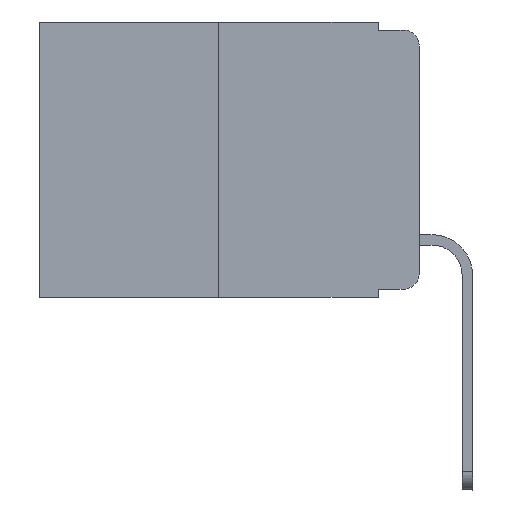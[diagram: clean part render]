
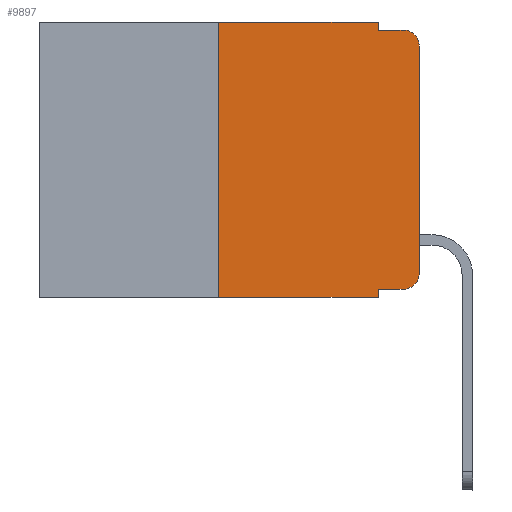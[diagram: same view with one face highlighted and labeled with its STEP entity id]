
A CAD part, left-side view. The second image highlights one B-rep face of the part: STEP entity #9897.
In plain terms, the highlighted planar face has unit normal (-1, 0, 0).
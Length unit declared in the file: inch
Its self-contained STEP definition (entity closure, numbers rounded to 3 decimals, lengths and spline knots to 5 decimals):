
#70 = DIRECTION ( 'NONE',  ( 0., 0., -1. ) ) ;
#277 = VERTEX_POINT ( 'NONE', #10054 ) ;
#329 = LINE ( 'NONE', #1274, #8766 ) ;
#504 = CARTESIAN_POINT ( 'NONE',  ( 0., 0.051, -0.333 ) ) ;
#809 = ORIENTED_EDGE ( 'NONE', *, *, #3885, .T. ) ;
#959 = LINE ( 'NONE', #3581, #6711 ) ;
#1002 = CARTESIAN_POINT ( 'NONE',  ( 0., 0.02, -0.01 ) ) ;
#1059 = VERTEX_POINT ( 'NONE', #4307 ) ;
#1081 = DIRECTION ( 'NONE',  ( 0., -1., 0. ) ) ;
#1229 = LINE ( 'NONE', #7632, #9691 ) ;
#1274 = CARTESIAN_POINT ( 'NONE',  ( 0., 0.051, 0. ) ) ;
#1391 = DIRECTION ( 'NONE',  ( 1., 0., 0. ) ) ;
#1441 = CARTESIAN_POINT ( 'NONE',  ( 0., 0.051, -0.333 ) ) ;
#1515 = EDGE_CURVE ( 'NONE', #10749, #10752, #8075, .T. ) ;
#1640 = ORIENTED_EDGE ( 'NONE', *, *, #2505, .F. ) ;
#1793 = ORIENTED_EDGE ( 'NONE', *, *, #2045, .T. ) ;
#1835 = CARTESIAN_POINT ( 'NONE',  ( 0., 0., -0.03 ) ) ;
#1882 = EDGE_LOOP ( 'NONE', ( #5099, #2190, #9951, #11490, #10899, #3770, #1793, #1640, #809, #9549 ) ) ;
#2009 = DIRECTION ( 'NONE',  ( 0., 0., -1. ) ) ;
#2045 = EDGE_CURVE ( 'NONE', #7577, #7876, #5255, .T. ) ;
#2190 = ORIENTED_EDGE ( 'NONE', *, *, #1515, .T. ) ;
#2258 = LINE ( 'NONE', #504, #5525 ) ;
#2370 = CARTESIAN_POINT ( 'NONE',  ( 0., 0.051, -0.343 ) ) ;
#2505 = EDGE_CURVE ( 'NONE', #11327, #7876, #9865, .T. ) ;
#2786 = CARTESIAN_POINT ( 'NONE',  ( 0., 0.051, -0.01 ) ) ;
#2829 = DIRECTION ( 'NONE',  ( 0., 0., -1. ) ) ;
#2870 = VECTOR ( 'NONE', #6007, 39.37008 ) ;
#3147 = PLANE ( 'NONE',  #6907 ) ;
#3581 = CARTESIAN_POINT ( 'NONE',  ( 0., 0., 0. ) ) ;
#3628 = CARTESIAN_POINT ( 'NONE',  ( 0., 0.051, 0. ) ) ;
#3770 = ORIENTED_EDGE ( 'NONE', *, *, #8933, .F. ) ;
#3787 = CARTESIAN_POINT ( 'NONE',  ( 0., 0.25, -0.343 ) ) ;
#3885 = EDGE_CURVE ( 'NONE', #11327, #277, #2258, .T. ) ;
#4074 = DIRECTION ( 'NONE',  ( 0., -1., 0. ) ) ;
#4307 = CARTESIAN_POINT ( 'NONE',  ( 0., 0.25, 0. ) ) ;
#4367 = EDGE_CURVE ( 'NONE', #10366, #10752, #10972, .T. ) ;
#4711 = EDGE_CURVE ( 'NONE', #277, #7251, #8135, .T. ) ;
#4944 = CARTESIAN_POINT ( 'NONE',  ( 0., 0.051, 0. ) ) ;
#5099 = ORIENTED_EDGE ( 'NONE', *, *, #9207, .T. ) ;
#5255 = LINE ( 'NONE', #6184, #10848 ) ;
#5421 = DIRECTION ( 'NONE',  ( 0., 0., 1. ) ) ;
#5525 = VECTOR ( 'NONE', #4074, 39.37008 ) ;
#5894 = CARTESIAN_POINT ( 'NONE',  ( 0., 0.473, 0. ) ) ;
#6007 = DIRECTION ( 'NONE',  ( 0., -1., 0. ) ) ;
#6184 = CARTESIAN_POINT ( 'NONE',  ( 0., 0.473, -0.343 ) ) ;
#6367 = DIRECTION ( 'NONE',  ( -1., 0., 0. ) ) ;
#6380 = DIRECTION ( 'NONE',  ( 0., -1., 0. ) ) ;
#6408 = CARTESIAN_POINT ( 'NONE',  ( 0., 0.02, -0.03 ) ) ;
#6418 = CARTESIAN_POINT ( 'NONE',  ( 0., 0., -0.313 ) ) ;
#6455 = EDGE_CURVE ( 'NONE', #1059, #9438, #7382, .T. ) ;
#6711 = VECTOR ( 'NONE', #5421, 39.37008 ) ;
#6907 = AXIS2_PLACEMENT_3D ( 'NONE', #7692, #1391, #9592 ) ;
#7000 = AXIS2_PLACEMENT_3D ( 'NONE', #10849, #6367, #2829 ) ;
#7251 = VERTEX_POINT ( 'NONE', #6418 ) ;
#7382 = LINE ( 'NONE', #5894, #2870 ) ;
#7577 = VERTEX_POINT ( 'NONE', #3787 ) ;
#7632 = CARTESIAN_POINT ( 'NONE',  ( 0., 0.25, 0. ) ) ;
#7692 = CARTESIAN_POINT ( 'NONE',  ( 0., 0.473, 0. ) ) ;
#7758 = VECTOR ( 'NONE', #9752, 39.37008 ) ;
#7876 = VERTEX_POINT ( 'NONE', #2370 ) ;
#8075 = CIRCLE ( 'NONE', #8438, 0.02 ) ;
#8135 = CIRCLE ( 'NONE', #7000, 0.02 ) ;
#8438 = AXIS2_PLACEMENT_3D ( 'NONE', #6408, #11000, #2009 ) ;
#8474 = CARTESIAN_POINT ( 'NONE',  ( 0., 0.051, -0.01 ) ) ;
#8658 = EDGE_CURVE ( 'NONE', #9438, #10366, #329, .T. ) ;
#8766 = VECTOR ( 'NONE', #70, 39.37008 ) ;
#8801 = FACE_OUTER_BOUND ( 'NONE', #1882, .T. ) ;
#8933 = EDGE_CURVE ( 'NONE', #7577, #1059, #1229, .T. ) ;
#9207 = EDGE_CURVE ( 'NONE', #7251, #10749, #959, .T. ) ;
#9328 = VECTOR ( 'NONE', #6380, 39.37008 ) ;
#9438 = VERTEX_POINT ( 'NONE', #4944 ) ;
#9549 = ORIENTED_EDGE ( 'NONE', *, *, #4711, .T. ) ;
#9592 = DIRECTION ( 'NONE',  ( 0., 0., -1. ) ) ;
#9691 = VECTOR ( 'NONE', #11209, 39.37008 ) ;
#9752 = DIRECTION ( 'NONE',  ( 0., 0., -1. ) ) ;
#9865 = LINE ( 'NONE', #3628, #7758 ) ;
#9897 = ADVANCED_FACE ( 'NONE', ( #8801 ), #3147, .F. ) ;
#9951 = ORIENTED_EDGE ( 'NONE', *, *, #4367, .F. ) ;
#10054 = CARTESIAN_POINT ( 'NONE',  ( 0., 0.02, -0.333 ) ) ;
#10366 = VERTEX_POINT ( 'NONE', #8474 ) ;
#10749 = VERTEX_POINT ( 'NONE', #1835 ) ;
#10752 = VERTEX_POINT ( 'NONE', #1002 ) ;
#10848 = VECTOR ( 'NONE', #1081, 39.37008 ) ;
#10849 = CARTESIAN_POINT ( 'NONE',  ( 0., 0.02, -0.313 ) ) ;
#10899 = ORIENTED_EDGE ( 'NONE', *, *, #6455, .F. ) ;
#10972 = LINE ( 'NONE', #2786, #9328 ) ;
#11000 = DIRECTION ( 'NONE',  ( -1., 0., 0. ) ) ;
#11209 = DIRECTION ( 'NONE',  ( 0., 0., 1. ) ) ;
#11327 = VERTEX_POINT ( 'NONE', #1441 ) ;
#11490 = ORIENTED_EDGE ( 'NONE', *, *, #8658, .F. ) ;
